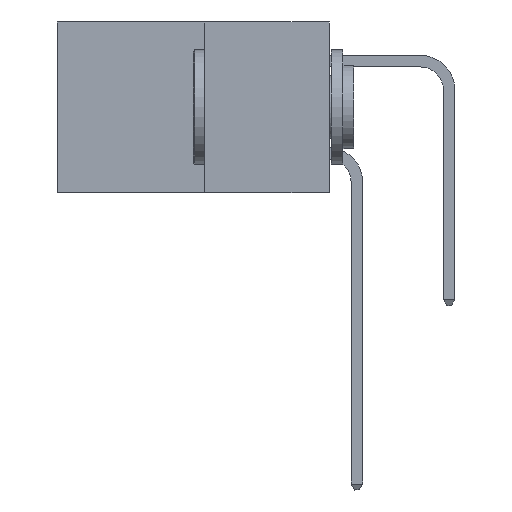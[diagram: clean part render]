
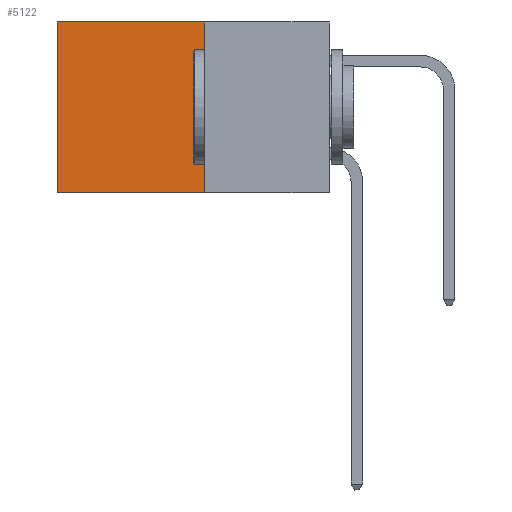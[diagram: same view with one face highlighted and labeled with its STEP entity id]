
A CAD part, left-side view. The second image highlights one B-rep face of the part: STEP entity #5122.
In plain terms, the highlighted planar face has unit normal (-1, 0, 0).
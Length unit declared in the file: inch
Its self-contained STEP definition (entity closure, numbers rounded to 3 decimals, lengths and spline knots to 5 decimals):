
#10 = LINE ( 'NONE', #24105, #24517 ) ;
#995 = ORIENTED_EDGE ( 'NONE', *, *, #17043, .F. ) ;
#1296 = ORIENTED_EDGE ( 'NONE', *, *, #22612, .T. ) ;
#2659 = VECTOR ( 'NONE', #17700, 39.37008 ) ;
#3949 = DIRECTION ( 'NONE',  ( 0., 1., 0. ) ) ;
#5122 = ADVANCED_FACE ( 'NONE', ( #25508 ), #13230, .F. ) ;
#8141 = VERTEX_POINT ( 'NONE', #31762 ) ;
#9435 = VECTOR ( 'NONE', #29045, 39.37008 ) ;
#9480 = AXIS2_PLACEMENT_3D ( 'NONE', #13188, #17350, #17339 ) ;
#9763 = EDGE_CURVE ( 'NONE', #15247, #11923, #22861, .T. ) ;
#10788 = EDGE_LOOP ( 'NONE', ( #27854, #995, #11397, #1296 ) ) ;
#11108 = DIRECTION ( 'NONE',  ( 0., 1., 0. ) ) ;
#11397 = ORIENTED_EDGE ( 'NONE', *, *, #24231, .F. ) ;
#11466 = CARTESIAN_POINT ( 'NONE',  ( 0.277, 0.27, -0.37 ) ) ;
#11923 = VERTEX_POINT ( 'NONE', #26937 ) ;
#13188 = CARTESIAN_POINT ( 'NONE',  ( 0.277, 0.27, -0.37 ) ) ;
#13230 = PLANE ( 'NONE',  #9480 ) ;
#15247 = VERTEX_POINT ( 'NONE', #28811 ) ;
#17043 = EDGE_CURVE ( 'NONE', #8141, #11923, #10, .T. ) ;
#17339 = DIRECTION ( 'NONE',  ( 0., 0., -1. ) ) ;
#17350 = DIRECTION ( 'NONE',  ( 1., 0., 0. ) ) ;
#17700 = DIRECTION ( 'NONE',  ( 0., 0., -1. ) ) ;
#22612 = EDGE_CURVE ( 'NONE', #29737, #15247, #24232, .T. ) ;
#22861 = LINE ( 'NONE', #27614, #2659 ) ;
#23792 = CARTESIAN_POINT ( 'NONE',  ( 0.277, 0.27, 0. ) ) ;
#24105 = CARTESIAN_POINT ( 'NONE',  ( 0.277, 0.27, -0.37 ) ) ;
#24231 = EDGE_CURVE ( 'NONE', #29737, #8141, #29461, .T. ) ;
#24232 = LINE ( 'NONE', #23792, #29932 ) ;
#24517 = VECTOR ( 'NONE', #3949, 39.37008 ) ;
#25287 = CARTESIAN_POINT ( 'NONE',  ( 0.277, 0.27, 0. ) ) ;
#25508 = FACE_OUTER_BOUND ( 'NONE', #10788, .T. ) ;
#26937 = CARTESIAN_POINT ( 'NONE',  ( 0.277, 0.59, -0.37 ) ) ;
#27614 = CARTESIAN_POINT ( 'NONE',  ( 0.277, 0.59, -0.37 ) ) ;
#27854 = ORIENTED_EDGE ( 'NONE', *, *, #9763, .T. ) ;
#28811 = CARTESIAN_POINT ( 'NONE',  ( 0.277, 0.59, 0. ) ) ;
#29045 = DIRECTION ( 'NONE',  ( 0., 0., -1. ) ) ;
#29461 = LINE ( 'NONE', #11466, #9435 ) ;
#29737 = VERTEX_POINT ( 'NONE', #25287 ) ;
#29932 = VECTOR ( 'NONE', #11108, 39.37008 ) ;
#31762 = CARTESIAN_POINT ( 'NONE',  ( 0.277, 0.27, -0.37 ) ) ;
